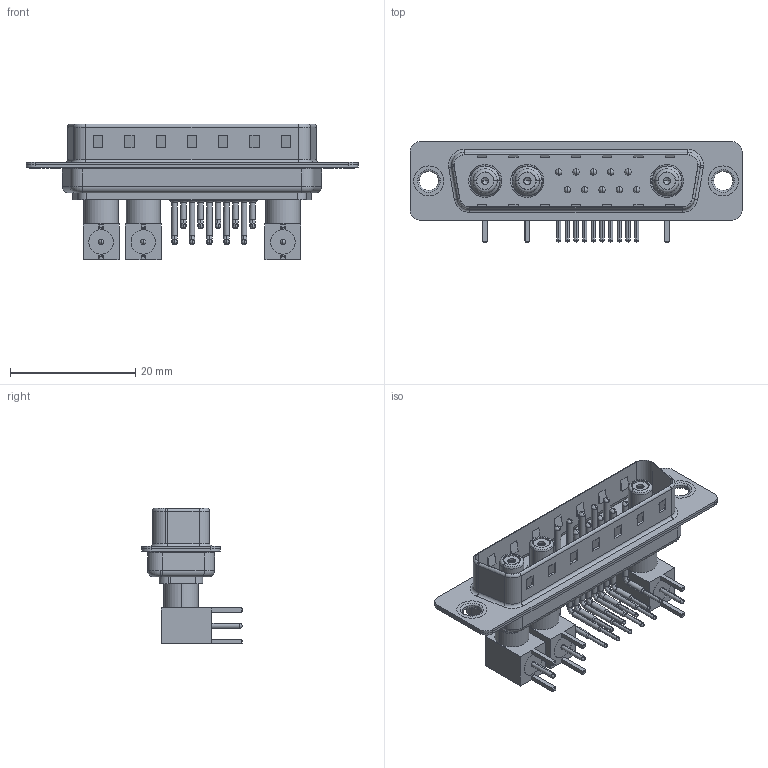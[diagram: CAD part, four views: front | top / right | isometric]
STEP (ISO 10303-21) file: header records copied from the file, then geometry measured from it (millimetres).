
FILE_DESCRIPTION (( 'STEP AP203' ), '1' );
FILE_NAME ('629-13W3240-7N1.STEP', '2022-05-10T02:35:34', ( '' ), ( '' ), 'SwSTEP 2.0', 'SolidWorks 2020', '' );
FILE_SCHEMA (( 'CONFIG_CONTROL_DESIGN' ));
Length unit declared in the file: millimetre
Products named in the file (17): Co-Ax Jack Assy_RA; 629Combo Shell Front_25 Contacts; 629-13W3240-7N1; Socket_RA; Locking Collar; 629Combo Thru Hole Rivet; Insulator RA Pin; 629Combo Shell Rear_25 Contacts; Insulator Socket 2; 629Combo Contact Row 1; 629Combo Housing_13W3; Insulator Socket; RA Back Shell; Co-Ax Jack_RA PC Tail; 629Combo Contact Row 2
Assembly tree (39 placements, depth 3):
  629-13W3240-7N1
    629Combo Housing_13W3
    629Combo Shell Rear_25 Contacts
    629Combo Shell Front_25 Contacts
    629Combo Thru Hole Rivet  x2
    Co-Ax Jack Assy_RA
      Co-Ax Jack_RA PC Tail
      Insulator Socket
      Insulator Socket 2
      Locking Collar
      Socket_RA
      RA Back Shell
      Insulator RA Pin
    Co-Ax Jack Assy_RA
      Co-Ax Jack_RA PC Tail
      Insulator Socket
      Insulator Socket 2
      Locking Collar
      Socket_RA
      RA Back Shell
      Insulator RA Pin
    Co-Ax Jack Assy_RA
      Co-Ax Jack_RA PC Tail
      Insulator Socket
      Insulator Socket 2
      Locking Collar
      Socket_RA
      RA Back Shell
      Insulator RA Pin
    629Combo Contact Row 1  x5
    629Combo Contact Row 2  x5
Bounding box: 53.05 x 16 x 21.71 mm (x, y, z)
Volume: 3577.6 mm3; surface area: 9759.1 mm2
Topology: 36 solids, 36 shells, 1906 faces, 5020 edges, 3215 vertices
Faces by surface type: plane 982, cylinder 682, cone 97, torus 76, bspline 63, sphere 6
Entity records: 26314 total; most frequent: CARTESIAN_POINT 4461, DIRECTION 4273, ORIENTED_EDGE 3900, EDGE_CURVE 1950, AXIS2_PLACEMENT_3D 1548, VERTEX_POINT 1251, VECTOR 1177, LINE 1177
